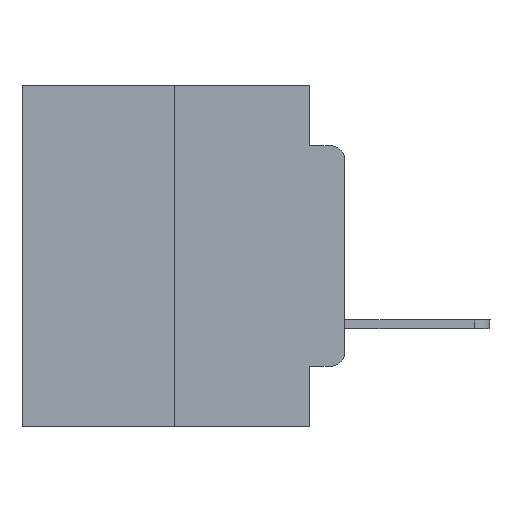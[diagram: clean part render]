
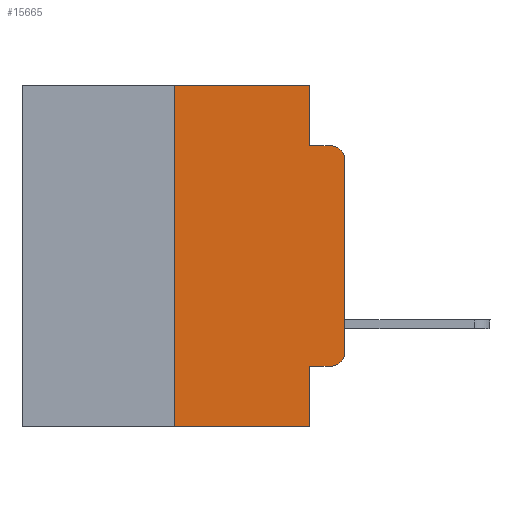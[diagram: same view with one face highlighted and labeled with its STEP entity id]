
A CAD part, left-side view. The second image highlights one B-rep face of the part: STEP entity #15665.
In plain terms, the highlighted planar face has unit normal (-1, 0, 0).
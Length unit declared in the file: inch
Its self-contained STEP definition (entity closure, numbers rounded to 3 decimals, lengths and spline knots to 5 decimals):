
#617 = ORIENTED_EDGE ( 'NONE', *, *, #13192, .F. ) ;
#1395 = VECTOR ( 'NONE', #4642, 39.37008 ) ;
#1446 = EDGE_CURVE ( 'NONE', #22740, #2914, #15710, .T. ) ;
#2164 = CARTESIAN_POINT ( 'NONE',  ( 0., 0.473, 0. ) ) ;
#2444 = CARTESIAN_POINT ( 'NONE',  ( 0., 0.25, 0. ) ) ;
#2914 = VERTEX_POINT ( 'NONE', #12968 ) ;
#3260 = CARTESIAN_POINT ( 'NONE',  ( 0., 0.051, -0.4115 ) ) ;
#3357 = LINE ( 'NONE', #12247, #15615 ) ;
#3686 = VECTOR ( 'NONE', #9739, 39.37008 ) ;
#3695 = CARTESIAN_POINT ( 'NONE',  ( 0., 0.02, -0.1085 ) ) ;
#4047 = EDGE_CURVE ( 'NONE', #8982, #22740, #20336, .T. ) ;
#4418 = ORIENTED_EDGE ( 'NONE', *, *, #14423, .F. ) ;
#4450 = VECTOR ( 'NONE', #13375, 39.37008 ) ;
#4642 = DIRECTION ( 'NONE',  ( 0., -1., 0. ) ) ;
#4807 = CARTESIAN_POINT ( 'NONE',  ( 0., 0.051, -0.5 ) ) ;
#4936 = EDGE_CURVE ( 'NONE', #23999, #18901, #3357, .T. ) ;
#5157 = VERTEX_POINT ( 'NONE', #8548 ) ;
#5445 = LINE ( 'NONE', #3260, #4450 ) ;
#5789 = EDGE_CURVE ( 'NONE', #18367, #23999, #20546, .T. ) ;
#5819 = ORIENTED_EDGE ( 'NONE', *, *, #10367, .T. ) ;
#5850 = CARTESIAN_POINT ( 'NONE',  ( 0., 0.473, 0. ) ) ;
#6056 = EDGE_CURVE ( 'NONE', #5157, #11052, #7479, .T. ) ;
#6398 = DIRECTION ( 'NONE',  ( 0., 0., -1. ) ) ;
#6625 = ORIENTED_EDGE ( 'NONE', *, *, #8276, .T. ) ;
#7479 = LINE ( 'NONE', #17548, #16086 ) ;
#7773 = PLANE ( 'NONE',  #22253 ) ;
#8276 = EDGE_CURVE ( 'NONE', #21184, #11052, #17319, .T. ) ;
#8548 = CARTESIAN_POINT ( 'NONE',  ( 0., 0.051, -0.4115 ) ) ;
#8982 = VERTEX_POINT ( 'NONE', #24730 ) ;
#9222 = ORIENTED_EDGE ( 'NONE', *, *, #1446, .T. ) ;
#9671 = CARTESIAN_POINT ( 'NONE',  ( 0., 0.02, -0.0885 ) ) ;
#9739 = DIRECTION ( 'NONE',  ( 0., 0., 1. ) ) ;
#9876 = CIRCLE ( 'NONE', #15513, 0.02 ) ;
#9979 = VERTEX_POINT ( 'NONE', #9671 ) ;
#10367 = EDGE_CURVE ( 'NONE', #5157, #8982, #5445, .T. ) ;
#10597 = ORIENTED_EDGE ( 'NONE', *, *, #5789, .F. ) ;
#11052 = VERTEX_POINT ( 'NONE', #4807 ) ;
#11517 = CARTESIAN_POINT ( 'NONE',  ( 0., 0., 0. ) ) ;
#12247 = CARTESIAN_POINT ( 'NONE',  ( 0., 0.051, 0. ) ) ;
#12418 = CARTESIAN_POINT ( 'NONE',  ( 0., 0.051, -0.0885 ) ) ;
#12456 = DIRECTION ( 'NONE',  ( 0., 0., -1. ) ) ;
#12649 = VECTOR ( 'NONE', #14181, 39.37008 ) ;
#12947 = CARTESIAN_POINT ( 'NONE',  ( 0., 0.25, 0. ) ) ;
#12955 = LINE ( 'NONE', #2444, #18528 ) ;
#12968 = CARTESIAN_POINT ( 'NONE',  ( 0., 0., -0.1085 ) ) ;
#13151 = CARTESIAN_POINT ( 'NONE',  ( 0., 0.25, -0.5 ) ) ;
#13192 = EDGE_CURVE ( 'NONE', #21184, #18367, #12955, .T. ) ;
#13375 = DIRECTION ( 'NONE',  ( 0., -1., 0. ) ) ;
#13404 = DIRECTION ( 'NONE',  ( 0., 0., -1. ) ) ;
#14130 = EDGE_CURVE ( 'NONE', #2914, #9979, #9876, .T. ) ;
#14132 = LINE ( 'NONE', #22400, #20804 ) ;
#14181 = DIRECTION ( 'NONE',  ( 0., -1., 0. ) ) ;
#14283 = ORIENTED_EDGE ( 'NONE', *, *, #4936, .F. ) ;
#14423 = EDGE_CURVE ( 'NONE', #18901, #9979, #14132, .T. ) ;
#14460 = CARTESIAN_POINT ( 'NONE',  ( 0., 0., -0.3915 ) ) ;
#15374 = DIRECTION ( 'NONE',  ( 0., 0., -1. ) ) ;
#15513 = AXIS2_PLACEMENT_3D ( 'NONE', #3695, #26836, #12456 ) ;
#15615 = VECTOR ( 'NONE', #22269, 39.37008 ) ;
#15665 = ADVANCED_FACE ( 'NONE', ( #26377 ), #7773, .F. ) ;
#15710 = LINE ( 'NONE', #11517, #3686 ) ;
#16086 = VECTOR ( 'NONE', #15374, 39.37008 ) ;
#16266 = ORIENTED_EDGE ( 'NONE', *, *, #14130, .T. ) ;
#16932 = EDGE_LOOP ( 'NONE', ( #9222, #16266, #4418, #14283, #10597, #617, #6625, #24891, #5819, #18260 ) ) ;
#17319 = LINE ( 'NONE', #23292, #1395 ) ;
#17548 = CARTESIAN_POINT ( 'NONE',  ( 0., 0.051, 0. ) ) ;
#17881 = CARTESIAN_POINT ( 'NONE',  ( 0., 0.02, -0.3915 ) ) ;
#18260 = ORIENTED_EDGE ( 'NONE', *, *, #4047, .T. ) ;
#18336 = DIRECTION ( 'NONE',  ( 0., -1., 0. ) ) ;
#18367 = VERTEX_POINT ( 'NONE', #12947 ) ;
#18528 = VECTOR ( 'NONE', #21224, 39.37008 ) ;
#18901 = VERTEX_POINT ( 'NONE', #12418 ) ;
#20336 = CIRCLE ( 'NONE', #24241, 0.02 ) ;
#20546 = LINE ( 'NONE', #5850, #12649 ) ;
#20709 = CARTESIAN_POINT ( 'NONE',  ( 0., 0.051, 0. ) ) ;
#20804 = VECTOR ( 'NONE', #18336, 39.37008 ) ;
#21184 = VERTEX_POINT ( 'NONE', #13151 ) ;
#21224 = DIRECTION ( 'NONE',  ( 0., 0., 1. ) ) ;
#22253 = AXIS2_PLACEMENT_3D ( 'NONE', #2164, #23103, #6398 ) ;
#22269 = DIRECTION ( 'NONE',  ( 0., 0., -1. ) ) ;
#22400 = CARTESIAN_POINT ( 'NONE',  ( 0., 0.051, -0.0885 ) ) ;
#22740 = VERTEX_POINT ( 'NONE', #14460 ) ;
#23103 = DIRECTION ( 'NONE',  ( 1., 0., 0. ) ) ;
#23292 = CARTESIAN_POINT ( 'NONE',  ( 0., 0.473, -0.5 ) ) ;
#23999 = VERTEX_POINT ( 'NONE', #20709 ) ;
#24241 = AXIS2_PLACEMENT_3D ( 'NONE', #17881, #26145, #13404 ) ;
#24730 = CARTESIAN_POINT ( 'NONE',  ( 0., 0.02, -0.4115 ) ) ;
#24891 = ORIENTED_EDGE ( 'NONE', *, *, #6056, .F. ) ;
#26145 = DIRECTION ( 'NONE',  ( -1., 0., 0. ) ) ;
#26377 = FACE_OUTER_BOUND ( 'NONE', #16932, .T. ) ;
#26836 = DIRECTION ( 'NONE',  ( -1., 0., 0. ) ) ;
